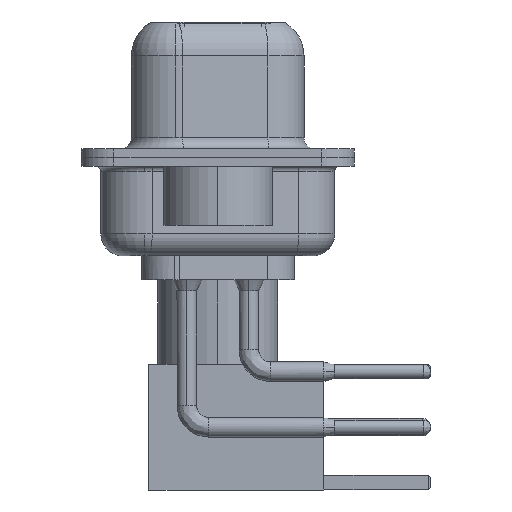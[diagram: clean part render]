
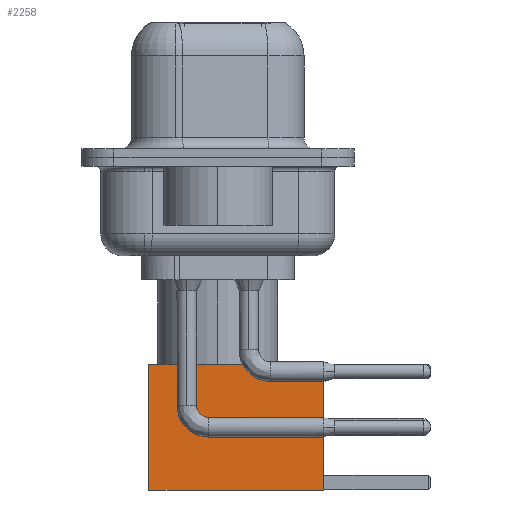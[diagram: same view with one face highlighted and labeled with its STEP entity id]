
A CAD part, left-side view. The second image highlights one B-rep face of the part: STEP entity #2258.
In plain terms, the highlighted face is planar.
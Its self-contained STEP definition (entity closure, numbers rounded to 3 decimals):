
#1030 = EDGE_CURVE ( 'NONE', #7428, #3527, #21176, .T. ) ;
#1064 = EDGE_LOOP ( 'NONE', ( #20136, #5544, #16895, #24394 ) ) ;
#1627 = PLANE ( 'NONE',  #20725 ) ;
#1756 = LINE ( 'NONE', #3607, #4466 ) ;
#1887 = CARTESIAN_POINT ( 'NONE',  ( -2.875, 2.875, 0. ) ) ;
#2258 = ADVANCED_FACE ( 'NONE', ( #13523 ), #1627, .T. ) ;
#3281 = CARTESIAN_POINT ( 'NONE',  ( 0., 2.875, 0. ) ) ;
#3527 = VERTEX_POINT ( 'NONE', #1887 ) ;
#3565 = DIRECTION ( 'NONE',  ( -1., 0., 0. ) ) ;
#3607 = CARTESIAN_POINT ( 'NONE',  ( -2.875, 2.875, 0. ) ) ;
#3851 = DIRECTION ( 'NONE',  ( 0., 1., 0. ) ) ;
#4466 = VECTOR ( 'NONE', #15606, 1000. ) ;
#5544 = ORIENTED_EDGE ( 'NONE', *, *, #1030, .T. ) ;
#7428 = VERTEX_POINT ( 'NONE', #25230 ) ;
#7872 = CARTESIAN_POINT ( 'NONE',  ( 0., 2.875, 8. ) ) ;
#8492 = VECTOR ( 'NONE', #24582, 1000. ) ;
#8524 = VECTOR ( 'NONE', #11395, 1000. ) ;
#8826 = VERTEX_POINT ( 'NONE', #19003 ) ;
#10639 = CARTESIAN_POINT ( 'NONE',  ( 2.875, 2.875, 0. ) ) ;
#10673 = EDGE_CURVE ( 'NONE', #8826, #22343, #21465, .T. ) ;
#10952 = EDGE_CURVE ( 'NONE', #8826, #7428, #16612, .T. ) ;
#11395 = DIRECTION ( 'NONE',  ( -1., 0., 0. ) ) ;
#13523 = FACE_OUTER_BOUND ( 'NONE', #1064, .T. ) ;
#14270 = VECTOR ( 'NONE', #3565, 1000. ) ;
#15606 = DIRECTION ( 'NONE',  ( 0., 0., -1. ) ) ;
#16612 = LINE ( 'NONE', #10639, #8492 ) ;
#16895 = ORIENTED_EDGE ( 'NONE', *, *, #23161, .F. ) ;
#17986 = CARTESIAN_POINT ( 'NONE',  ( -2.875, 2.875, 8. ) ) ;
#19003 = CARTESIAN_POINT ( 'NONE',  ( 2.875, 2.875, 8. ) ) ;
#20136 = ORIENTED_EDGE ( 'NONE', *, *, #10952, .T. ) ;
#20725 = AXIS2_PLACEMENT_3D ( 'NONE', #23700, #3851, #21756 ) ;
#21176 = LINE ( 'NONE', #3281, #8524 ) ;
#21465 = LINE ( 'NONE', #7872, #14270 ) ;
#21756 = DIRECTION ( 'NONE',  ( 0., 0., 1. ) ) ;
#22343 = VERTEX_POINT ( 'NONE', #17986 ) ;
#23161 = EDGE_CURVE ( 'NONE', #22343, #3527, #1756, .T. ) ;
#23700 = CARTESIAN_POINT ( 'NONE',  ( 2.875, 2.875, 0. ) ) ;
#24394 = ORIENTED_EDGE ( 'NONE', *, *, #10673, .F. ) ;
#24582 = DIRECTION ( 'NONE',  ( 0., 0., -1. ) ) ;
#25230 = CARTESIAN_POINT ( 'NONE',  ( 2.875, 2.875, 0. ) ) ;
